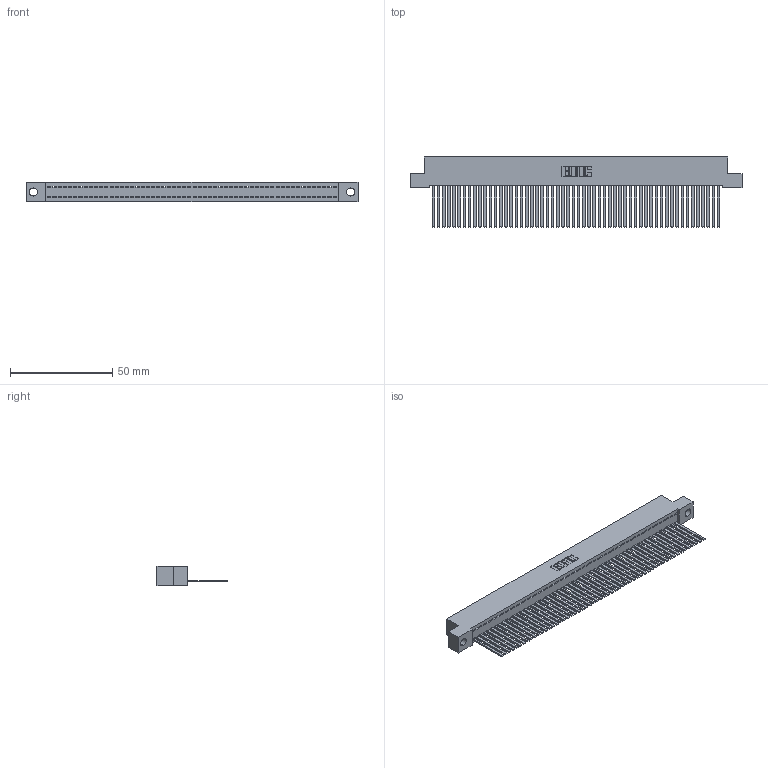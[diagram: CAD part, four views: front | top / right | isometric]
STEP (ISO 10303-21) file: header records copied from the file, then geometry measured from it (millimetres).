
FILE_DESCRIPTION (( 'STEP AP203' ), '1' );
FILE_NAME ('342-056-544-104.STEP', '2018-08-13T03:53:55', ( '' ), ( '' ), 'SwSTEP 2.0', 'SolidWorks 2016', '' );
FILE_SCHEMA (( 'CONFIG_CONTROL_DESIGN' ));
Length unit declared in the file: inch
Products named in the file (3): 342 Part_.156 TH; 345-292-001_345-293-144; 342-056-544-104
Assembly tree (57 placements, depth 2):
  342-056-544-104
    342 Part_.156 TH
    345-292-001_345-293-144  x56
Bounding box: 162.56 x 34.3 x 9.4 mm (x, y, z)
Volume: 14866.4 mm3; surface area: 23756.6 mm2
Topology: 57 solids, 57 shells, 3022 faces, 9147 edges, 6022 vertices
Faces by surface type: plane 2194, cylinder 828
Entity records: 32111 total; most frequent: CARTESIAN_POINT 5542, ORIENTED_EDGE 5534, DIRECTION 4643, EDGE_CURVE 2767, VECTOR 2643, LINE 2643, VERTEX_POINT 1842, AXIS2_PLACEMENT_3D 1000
